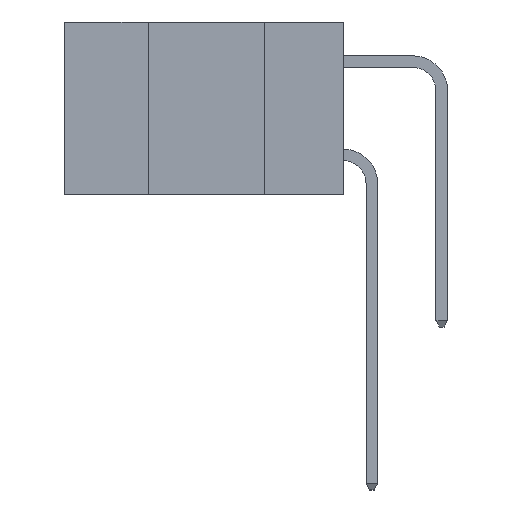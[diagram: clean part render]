
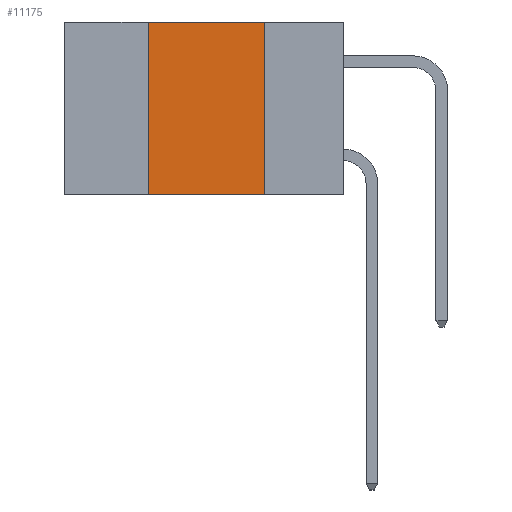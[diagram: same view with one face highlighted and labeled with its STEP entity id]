
A CAD part, left-side view. The second image highlights one B-rep face of the part: STEP entity #11175.
In plain terms, the highlighted planar face has unit normal (-1, 0, 0).
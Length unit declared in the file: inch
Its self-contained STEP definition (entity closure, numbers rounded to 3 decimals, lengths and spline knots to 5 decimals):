
#94 = CARTESIAN_POINT ( 'NONE',  ( 0., 0.42, -0.37 ) ) ;
#203 = CARTESIAN_POINT ( 'NONE',  ( 0., 0.6, 0. ) ) ;
#298 = CARTESIAN_POINT ( 'NONE',  ( 0., 0.17, -0.37 ) ) ;
#326 = LINE ( 'NONE', #12996, #2835 ) ;
#469 = LINE ( 'NONE', #8950, #10972 ) ;
#865 = DIRECTION ( 'NONE',  ( 0., 0., -1. ) ) ;
#1188 = DIRECTION ( 'NONE',  ( 0., 0., 1. ) ) ;
#1286 = PLANE ( 'NONE',  #12653 ) ;
#1444 = CARTESIAN_POINT ( 'NONE',  ( 0., 0.42, 0. ) ) ;
#1617 = VERTEX_POINT ( 'NONE', #11371 ) ;
#2187 = VERTEX_POINT ( 'NONE', #298 ) ;
#2332 = DIRECTION ( 'NONE',  ( 0., 0., -1. ) ) ;
#2835 = VECTOR ( 'NONE', #5167, 39.37008 ) ;
#3014 = ORIENTED_EDGE ( 'NONE', *, *, #7749, .T. ) ;
#3695 = FACE_OUTER_BOUND ( 'NONE', #8506, .T. ) ;
#4478 = VECTOR ( 'NONE', #6976, 39.37008 ) ;
#5167 = DIRECTION ( 'NONE',  ( 0., -1., 0. ) ) ;
#5629 = VERTEX_POINT ( 'NONE', #7675 ) ;
#6851 = ORIENTED_EDGE ( 'NONE', *, *, #12938, .F. ) ;
#6976 = DIRECTION ( 'NONE',  ( 0., -1., 0. ) ) ;
#7156 = LINE ( 'NONE', #10889, #4478 ) ;
#7675 = CARTESIAN_POINT ( 'NONE',  ( 0., 0.17, 0. ) ) ;
#7749 = EDGE_CURVE ( 'NONE', #1617, #2187, #7156, .T. ) ;
#7757 = ORIENTED_EDGE ( 'NONE', *, *, #11700, .F. ) ;
#7766 = VECTOR ( 'NONE', #1188, 39.37008 ) ;
#8401 = DIRECTION ( 'NONE',  ( 1., 0., 0. ) ) ;
#8506 = EDGE_LOOP ( 'NONE', ( #6851, #12048, #7757, #3014 ) ) ;
#8950 = CARTESIAN_POINT ( 'NONE',  ( 0., 0.17, -0.37 ) ) ;
#10889 = CARTESIAN_POINT ( 'NONE',  ( 0., 0.6, -0.37 ) ) ;
#10972 = VECTOR ( 'NONE', #865, 39.37008 ) ;
#11175 = ADVANCED_FACE ( 'NONE', ( #3695 ), #1286, .F. ) ;
#11371 = CARTESIAN_POINT ( 'NONE',  ( 0., 0.42, -0.37 ) ) ;
#11700 = EDGE_CURVE ( 'NONE', #1617, #11917, #12917, .T. ) ;
#11917 = VERTEX_POINT ( 'NONE', #1444 ) ;
#12048 = ORIENTED_EDGE ( 'NONE', *, *, #12320, .F. ) ;
#12320 = EDGE_CURVE ( 'NONE', #11917, #5629, #326, .T. ) ;
#12653 = AXIS2_PLACEMENT_3D ( 'NONE', #203, #8401, #2332 ) ;
#12917 = LINE ( 'NONE', #94, #7766 ) ;
#12938 = EDGE_CURVE ( 'NONE', #5629, #2187, #469, .T. ) ;
#12996 = CARTESIAN_POINT ( 'NONE',  ( 0., 0.6, 0. ) ) ;
